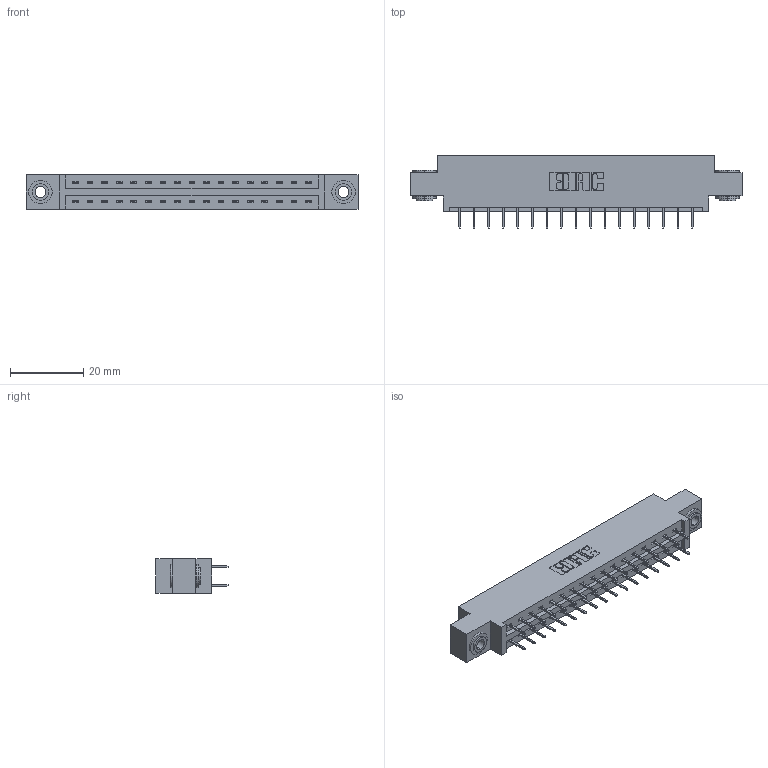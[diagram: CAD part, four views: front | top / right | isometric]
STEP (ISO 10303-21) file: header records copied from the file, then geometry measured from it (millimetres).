
FILE_DESCRIPTION (( 'STEP AP203' ), '1' );
FILE_NAME ('337-034-524-803.STEP', '2019-10-11T01:46:49', ( '' ), ( '' ), 'SwSTEP 2.0', 'SolidWorks 2016', '' );
FILE_SCHEMA (( 'CONFIG_CONTROL_DESIGN' ));
Length unit declared in the file: inch
Products named in the file (4): 337-034-524-803; 337 Part_0.170 Offset - 0.156 Dia-TH; 345-292-001_345-293-124; 345-250-002_345-250-002-102
Assembly tree (37 placements, depth 2):
  337-034-524-803
    337 Part_0.170 Offset - 0.156 Dia-TH
    345-292-001_345-293-124  x34
    345-250-002_345-250-002-102  x2
Bounding box: 90.37 x 19.69 x 9.4 mm (x, y, z)
Volume: 9041.9 mm3; surface area: 10151.9 mm2
Topology: 37 solids, 37 shells, 2128 faces, 6009 edges, 3866 vertices
Faces by surface type: plane 1580, cylinder 540, cone 8
Entity records: 17270 total; most frequent: CARTESIAN_POINT 2905, ORIENTED_EDGE 2834, DIRECTION 2551, EDGE_CURVE 1417, VECTOR 1269, LINE 1269, VERTEX_POINT 938, AXIS2_PLACEMENT_3D 641
